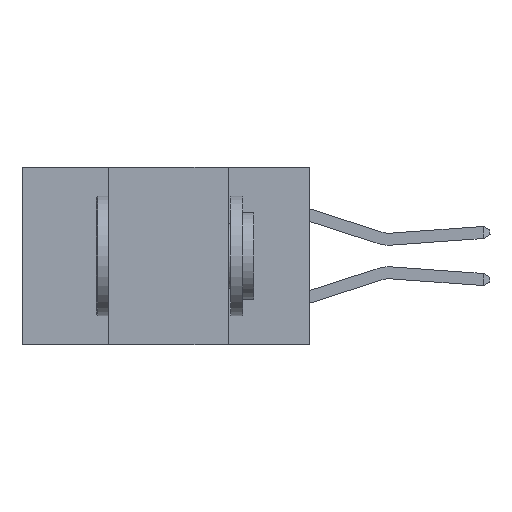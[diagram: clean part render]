
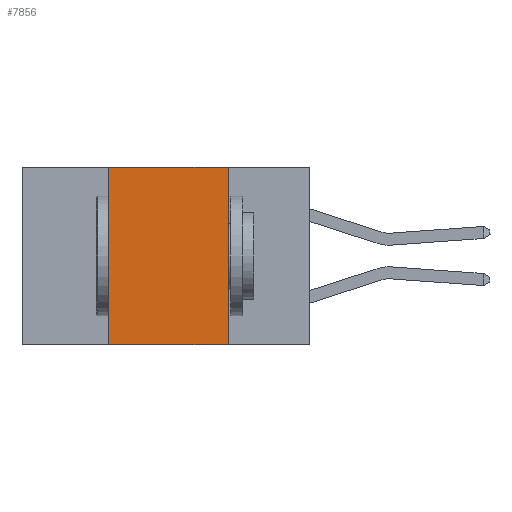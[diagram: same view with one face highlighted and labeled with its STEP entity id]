
A CAD part, left-side view. The second image highlights one B-rep face of the part: STEP entity #7856.
In plain terms, the highlighted planar face has unit normal (-1, 0, 0).
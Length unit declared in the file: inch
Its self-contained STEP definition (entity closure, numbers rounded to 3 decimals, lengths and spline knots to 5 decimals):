
#581 = DIRECTION ( 'NONE',  ( 0., 0., -1. ) ) ;
#638 = FACE_OUTER_BOUND ( 'NONE', #6657, .T. ) ;
#979 = EDGE_CURVE ( 'NONE', #10981, #9637, #1444, .T. ) ;
#1229 = ORIENTED_EDGE ( 'NONE', *, *, #6465, .T. ) ;
#1335 = CARTESIAN_POINT ( 'NONE',  ( 0., 0.42, -0.37 ) ) ;
#1444 = LINE ( 'NONE', #10250, #6561 ) ;
#4293 = CARTESIAN_POINT ( 'NONE',  ( 0., 0.42, 0. ) ) ;
#4304 = CARTESIAN_POINT ( 'NONE',  ( 0., 0.17, 0. ) ) ;
#4724 = AXIS2_PLACEMENT_3D ( 'NONE', #6460, #9459, #581 ) ;
#4737 = LINE ( 'NONE', #10410, #8801 ) ;
#5262 = CARTESIAN_POINT ( 'NONE',  ( 0., 0.6, 0. ) ) ;
#5767 = DIRECTION ( 'NONE',  ( 0., 0., -1. ) ) ;
#6079 = ORIENTED_EDGE ( 'NONE', *, *, #9214, .F. ) ;
#6218 = LINE ( 'NONE', #5262, #6364 ) ;
#6364 = VECTOR ( 'NONE', #8196, 39.37008 ) ;
#6460 = CARTESIAN_POINT ( 'NONE',  ( 0., 0.6, 0. ) ) ;
#6465 = EDGE_CURVE ( 'NONE', #10981, #9939, #10278, .T. ) ;
#6500 = ORIENTED_EDGE ( 'NONE', *, *, #10166, .F. ) ;
#6561 = VECTOR ( 'NONE', #8390, 39.37008 ) ;
#6657 = EDGE_LOOP ( 'NONE', ( #6500, #6079, #9696, #1229 ) ) ;
#7856 = ADVANCED_FACE ( 'NONE', ( #638 ), #11272, .F. ) ;
#8196 = DIRECTION ( 'NONE',  ( 0., -1., 0. ) ) ;
#8390 = DIRECTION ( 'NONE',  ( 0., 0., 1. ) ) ;
#8598 = VECTOR ( 'NONE', #11136, 39.37008 ) ;
#8801 = VECTOR ( 'NONE', #5767, 39.37008 ) ;
#8897 = CARTESIAN_POINT ( 'NONE',  ( 0., 0.17, -0.37 ) ) ;
#9138 = VERTEX_POINT ( 'NONE', #4304 ) ;
#9214 = EDGE_CURVE ( 'NONE', #9637, #9138, #6218, .T. ) ;
#9459 = DIRECTION ( 'NONE',  ( 1., 0., 0. ) ) ;
#9637 = VERTEX_POINT ( 'NONE', #4293 ) ;
#9696 = ORIENTED_EDGE ( 'NONE', *, *, #979, .F. ) ;
#9939 = VERTEX_POINT ( 'NONE', #8897 ) ;
#10166 = EDGE_CURVE ( 'NONE', #9138, #9939, #4737, .T. ) ;
#10250 = CARTESIAN_POINT ( 'NONE',  ( 0., 0.42, -0.37 ) ) ;
#10278 = LINE ( 'NONE', #11326, #8598 ) ;
#10410 = CARTESIAN_POINT ( 'NONE',  ( 0., 0.17, -0.37 ) ) ;
#10981 = VERTEX_POINT ( 'NONE', #1335 ) ;
#11136 = DIRECTION ( 'NONE',  ( 0., -1., 0. ) ) ;
#11272 = PLANE ( 'NONE',  #4724 ) ;
#11326 = CARTESIAN_POINT ( 'NONE',  ( 0., 0.6, -0.37 ) ) ;
